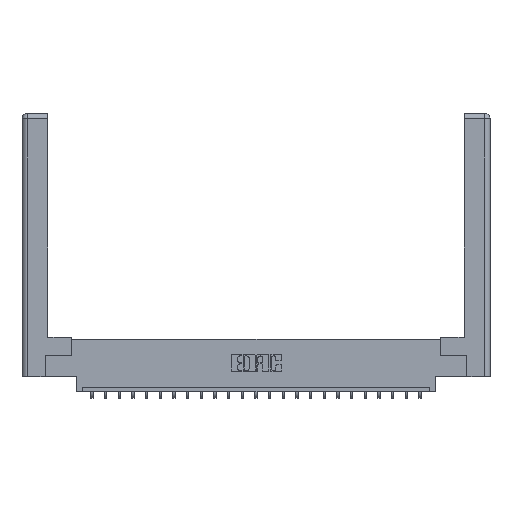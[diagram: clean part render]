
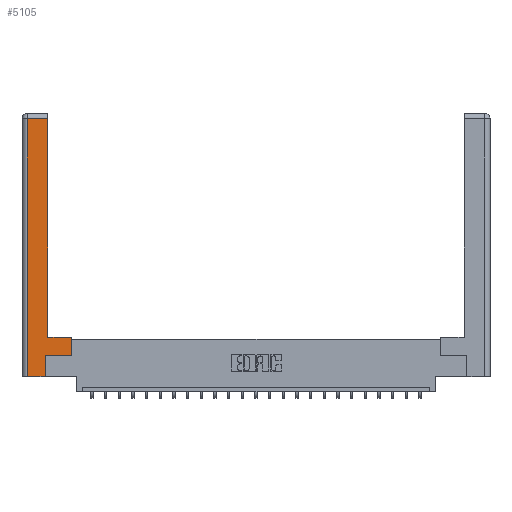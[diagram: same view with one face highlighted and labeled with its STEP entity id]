
A CAD part, top view. The second image highlights one B-rep face of the part: STEP entity #5105.
In plain terms, the highlighted planar face has unit normal (0, 0, 1).
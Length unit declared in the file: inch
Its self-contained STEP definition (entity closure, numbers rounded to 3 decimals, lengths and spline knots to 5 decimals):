
#244 = CARTESIAN_POINT ( 'NONE',  ( 0.565, 0.45, 0. ) ) ;
#424 = ORIENTED_EDGE ( 'NONE', *, *, #4865, .T. ) ;
#434 = PLANE ( 'NONE',  #13392 ) ;
#452 = CARTESIAN_POINT ( 'NONE',  ( 0.265, 0.245, 0. ) ) ;
#722 = VERTEX_POINT ( 'NONE', #3911 ) ;
#1229 = CARTESIAN_POINT ( 'NONE',  ( 0.0615, 2.94, 0. ) ) ;
#1230 = DIRECTION ( 'NONE',  ( 0., 1., 0. ) ) ;
#1287 = VERTEX_POINT ( 'NONE', #12976 ) ;
#1511 = CARTESIAN_POINT ( 'NONE',  ( 0.295, 0.45, 0. ) ) ;
#2002 = ORIENTED_EDGE ( 'NONE', *, *, #18600, .T. ) ;
#2774 = EDGE_CURVE ( 'NONE', #1287, #6057, #22781, .T. ) ;
#2911 = CARTESIAN_POINT ( 'NONE',  ( 0.565, 0.245, 0. ) ) ;
#3555 = DIRECTION ( 'NONE',  ( 0., 1., 0. ) ) ;
#3615 = LINE ( 'NONE', #1229, #6727 ) ;
#3911 = CARTESIAN_POINT ( 'NONE',  ( 0.565, 0.45, 0. ) ) ;
#4443 = VECTOR ( 'NONE', #13292, 39.37008 ) ;
#4865 = EDGE_CURVE ( 'NONE', #722, #1287, #13547, .T. ) ;
#5105 = ADVANCED_FACE ( 'NONE', ( #5822 ), #434, .F. ) ;
#5556 = EDGE_CURVE ( 'NONE', #13361, #722, #5572, .T. ) ;
#5572 = LINE ( 'NONE', #244, #12952 ) ;
#5624 = ORIENTED_EDGE ( 'NONE', *, *, #2774, .T. ) ;
#5672 = ORIENTED_EDGE ( 'NONE', *, *, #18050, .T. ) ;
#5822 = FACE_OUTER_BOUND ( 'NONE', #14581, .T. ) ;
#6057 = VERTEX_POINT ( 'NONE', #19918 ) ;
#6709 = LINE ( 'NONE', #2911, #11791 ) ;
#6727 = VECTOR ( 'NONE', #14041, 39.37008 ) ;
#7147 = VECTOR ( 'NONE', #9693, 39.37008 ) ;
#7359 = DIRECTION ( 'NONE',  ( 1., 0., 0. ) ) ;
#8048 = VERTEX_POINT ( 'NONE', #13820 ) ;
#8639 = VERTEX_POINT ( 'NONE', #452 ) ;
#8698 = EDGE_CURVE ( 'NONE', #11551, #22078, #16799, .T. ) ;
#8768 = CARTESIAN_POINT ( 'NONE',  ( 0.265, 0.245, 0. ) ) ;
#9262 = LINE ( 'NONE', #19936, #4443 ) ;
#9693 = DIRECTION ( 'NONE',  ( 0., -1., 0. ) ) ;
#10677 = CARTESIAN_POINT ( 'NONE',  ( 0.0615, 2.94, 0. ) ) ;
#11551 = VERTEX_POINT ( 'NONE', #10677 ) ;
#11791 = VECTOR ( 'NONE', #7359, 39.37008 ) ;
#11818 = VECTOR ( 'NONE', #14321, 39.37008 ) ;
#12952 = VECTOR ( 'NONE', #3555, 39.37008 ) ;
#12976 = CARTESIAN_POINT ( 'NONE',  ( 0.295, 0.45, 0. ) ) ;
#13292 = DIRECTION ( 'NONE',  ( 1., 0., 0. ) ) ;
#13361 = VERTEX_POINT ( 'NONE', #18574 ) ;
#13392 = AXIS2_PLACEMENT_3D ( 'NONE', #18643, #18733, #15098 ) ;
#13547 = LINE ( 'NONE', #1511, #11818 ) ;
#13820 = CARTESIAN_POINT ( 'NONE',  ( 0.265, 0., 0. ) ) ;
#14041 = DIRECTION ( 'NONE',  ( -1., 0., 0. ) ) ;
#14321 = DIRECTION ( 'NONE',  ( -1., 0., 0. ) ) ;
#14581 = EDGE_LOOP ( 'NONE', ( #5624, #5672, #18341, #2002, #20865, #15690, #19271, #424 ) ) ;
#15098 = DIRECTION ( 'NONE',  ( -1., 0., 0. ) ) ;
#15690 = ORIENTED_EDGE ( 'NONE', *, *, #18565, .T. ) ;
#16799 = LINE ( 'NONE', #20528, #7147 ) ;
#17283 = VECTOR ( 'NONE', #17648, 39.37008 ) ;
#17286 = EDGE_CURVE ( 'NONE', #8048, #8639, #18155, .T. ) ;
#17648 = DIRECTION ( 'NONE',  ( 0., 1., 0. ) ) ;
#18050 = EDGE_CURVE ( 'NONE', #6057, #11551, #3615, .T. ) ;
#18155 = LINE ( 'NONE', #8768, #17283 ) ;
#18197 = VECTOR ( 'NONE', #1230, 39.37008 ) ;
#18341 = ORIENTED_EDGE ( 'NONE', *, *, #8698, .T. ) ;
#18565 = EDGE_CURVE ( 'NONE', #8639, #13361, #6709, .T. ) ;
#18574 = CARTESIAN_POINT ( 'NONE',  ( 0.565, 0.245, 0. ) ) ;
#18600 = EDGE_CURVE ( 'NONE', #22078, #8048, #9262, .T. ) ;
#18643 = CARTESIAN_POINT ( 'NONE',  ( 0., 0., 0. ) ) ;
#18733 = DIRECTION ( 'NONE',  ( 0., 0., -1. ) ) ;
#19271 = ORIENTED_EDGE ( 'NONE', *, *, #5556, .T. ) ;
#19918 = CARTESIAN_POINT ( 'NONE',  ( 0.295, 2.94, 0. ) ) ;
#19936 = CARTESIAN_POINT ( 'NONE',  ( 0.265, 0., 0. ) ) ;
#20528 = CARTESIAN_POINT ( 'NONE',  ( 0.0615, 0., 0. ) ) ;
#20865 = ORIENTED_EDGE ( 'NONE', *, *, #17286, .T. ) ;
#20930 = CARTESIAN_POINT ( 'NONE',  ( 0.0615, 0., 0. ) ) ;
#22078 = VERTEX_POINT ( 'NONE', #20930 ) ;
#22781 = LINE ( 'NONE', #23136, #18197 ) ;
#23136 = CARTESIAN_POINT ( 'NONE',  ( 0.295, 3., 0. ) ) ;
